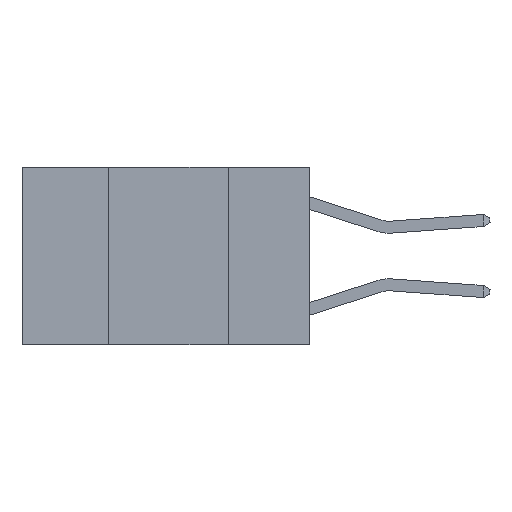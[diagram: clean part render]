
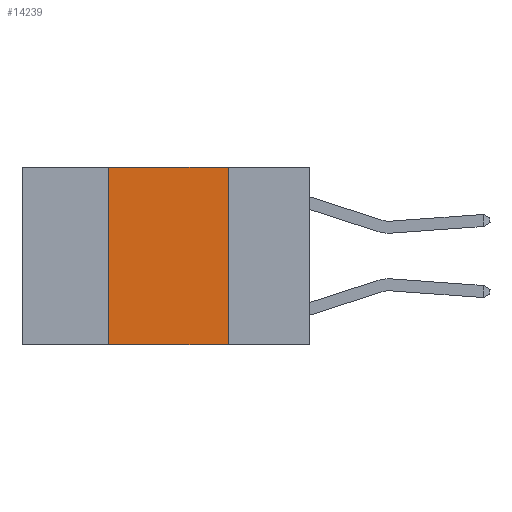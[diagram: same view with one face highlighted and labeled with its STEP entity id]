
A CAD part, left-side view. The second image highlights one B-rep face of the part: STEP entity #14239.
In plain terms, the highlighted planar face has unit normal (-1, 0, 0).
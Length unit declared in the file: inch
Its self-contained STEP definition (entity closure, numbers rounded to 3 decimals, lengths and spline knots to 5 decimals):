
#172 = CARTESIAN_POINT ( 'NONE',  ( 0., 0.6, -0.37 ) ) ;
#203 = LINE ( 'NONE', #7353, #5004 ) ;
#1248 = PLANE ( 'NONE',  #17056 ) ;
#1816 = ORIENTED_EDGE ( 'NONE', *, *, #11345, .F. ) ;
#2095 = VERTEX_POINT ( 'NONE', #6961 ) ;
#2354 = VERTEX_POINT ( 'NONE', #13517 ) ;
#2764 = EDGE_CURVE ( 'NONE', #2354, #17256, #15534, .T. ) ;
#3557 = VECTOR ( 'NONE', #15881, 39.37008 ) ;
#3709 = CARTESIAN_POINT ( 'NONE',  ( 0., 0.42, -0.37 ) ) ;
#4376 = LINE ( 'NONE', #13287, #22636 ) ;
#4687 = VERTEX_POINT ( 'NONE', #3709 ) ;
#4978 = EDGE_CURVE ( 'NONE', #4687, #17256, #7079, .T. ) ;
#5004 = VECTOR ( 'NONE', #18145, 39.37008 ) ;
#5398 = ORIENTED_EDGE ( 'NONE', *, *, #20395, .F. ) ;
#6380 = CARTESIAN_POINT ( 'NONE',  ( 0., 0.17, 0. ) ) ;
#6961 = CARTESIAN_POINT ( 'NONE',  ( 0., 0.42, 0. ) ) ;
#7079 = LINE ( 'NONE', #172, #3557 ) ;
#7353 = CARTESIAN_POINT ( 'NONE',  ( 0., 0.6, 0. ) ) ;
#7384 = CARTESIAN_POINT ( 'NONE',  ( 0., 0.17, -0.37 ) ) ;
#9770 = VECTOR ( 'NONE', #11911, 39.37008 ) ;
#10049 = EDGE_LOOP ( 'NONE', ( #19133, #1816, #5398, #21203 ) ) ;
#11345 = EDGE_CURVE ( 'NONE', #2095, #2354, #203, .T. ) ;
#11551 = DIRECTION ( 'NONE',  ( 0., 0., 1. ) ) ;
#11911 = DIRECTION ( 'NONE',  ( 0., 0., -1. ) ) ;
#13287 = CARTESIAN_POINT ( 'NONE',  ( 0., 0.42, 0. ) ) ;
#13455 = DIRECTION ( 'NONE',  ( 1., 0., 0. ) ) ;
#13517 = CARTESIAN_POINT ( 'NONE',  ( 0., 0.17, 0. ) ) ;
#13693 = FACE_OUTER_BOUND ( 'NONE', #10049, .T. ) ;
#14239 = ADVANCED_FACE ( 'NONE', ( #13693 ), #1248, .F. ) ;
#15534 = LINE ( 'NONE', #6380, #9770 ) ;
#15558 = CARTESIAN_POINT ( 'NONE',  ( 0., 0.6, 0. ) ) ;
#15881 = DIRECTION ( 'NONE',  ( 0., -1., 0. ) ) ;
#17056 = AXIS2_PLACEMENT_3D ( 'NONE', #15558, #13455, #17426 ) ;
#17256 = VERTEX_POINT ( 'NONE', #7384 ) ;
#17426 = DIRECTION ( 'NONE',  ( 0., 0., -1. ) ) ;
#18145 = DIRECTION ( 'NONE',  ( 0., -1., 0. ) ) ;
#19133 = ORIENTED_EDGE ( 'NONE', *, *, #2764, .F. ) ;
#20395 = EDGE_CURVE ( 'NONE', #4687, #2095, #4376, .T. ) ;
#21203 = ORIENTED_EDGE ( 'NONE', *, *, #4978, .T. ) ;
#22636 = VECTOR ( 'NONE', #11551, 39.37008 ) ;
